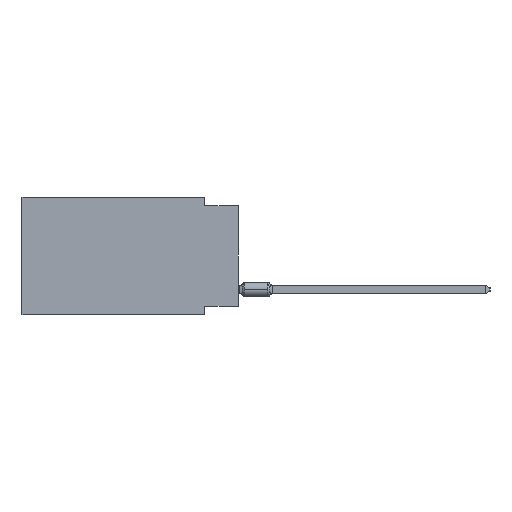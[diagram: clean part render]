
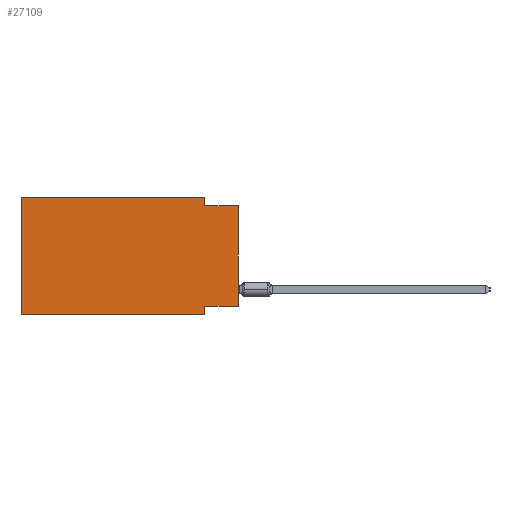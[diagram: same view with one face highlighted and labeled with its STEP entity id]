
A CAD part, left-side view. The second image highlights one B-rep face of the part: STEP entity #27109.
In plain terms, the highlighted planar face has unit normal (-1, 0, 0).
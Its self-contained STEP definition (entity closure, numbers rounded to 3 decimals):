
#609 = CARTESIAN_POINT ( 'NONE',  ( 0., 16.383, 0. ) ) ;
#1250 = LINE ( 'NONE', #60810, #87748 ) ;
#3824 = CARTESIAN_POINT ( 'NONE',  ( 0., 0., -0.635 ) ) ;
#5243 = LINE ( 'NONE', #35043, #7240 ) ;
#6862 = VECTOR ( 'NONE', #86803, 1000. ) ;
#7061 = EDGE_CURVE ( 'NONE', #28672, #7809, #38640, .T. ) ;
#7240 = VECTOR ( 'NONE', #81659, 1000. ) ;
#7387 = VERTEX_POINT ( 'NONE', #59777 ) ;
#7578 = DIRECTION ( 'NONE',  ( 0., 0., 1. ) ) ;
#7809 = VERTEX_POINT ( 'NONE', #36826 ) ;
#8173 = CARTESIAN_POINT ( 'NONE',  ( 0., 2.54, -8.255 ) ) ;
#9667 = LINE ( 'NONE', #47386, #38946 ) ;
#12269 = PLANE ( 'NONE',  #75564 ) ;
#12424 = ORIENTED_EDGE ( 'NONE', *, *, #78448, .F. ) ;
#12964 = VECTOR ( 'NONE', #28660, 1000. ) ;
#13235 = DIRECTION ( 'NONE',  ( 0., 0., -1. ) ) ;
#14143 = VERTEX_POINT ( 'NONE', #71076 ) ;
#15406 = CARTESIAN_POINT ( 'NONE',  ( 0., 2.54, 0. ) ) ;
#16245 = VERTEX_POINT ( 'NONE', #3824 ) ;
#27109 = ADVANCED_FACE ( 'NONE', ( #49978 ), #12269, .F. ) ;
#28228 = ORIENTED_EDGE ( 'NONE', *, *, #65236, .F. ) ;
#28518 = VERTEX_POINT ( 'NONE', #8173 ) ;
#28660 = DIRECTION ( 'NONE',  ( 0., 0., -1. ) ) ;
#28672 = VERTEX_POINT ( 'NONE', #40419 ) ;
#31737 = CARTESIAN_POINT ( 'NONE',  ( 0., 0., -8.255 ) ) ;
#33720 = LINE ( 'NONE', #78874, #6862 ) ;
#35043 = CARTESIAN_POINT ( 'NONE',  ( 0., 16.383, 0. ) ) ;
#36826 = CARTESIAN_POINT ( 'NONE',  ( 0., 2.54, -8.89 ) ) ;
#37214 = EDGE_CURVE ( 'NONE', #7387, #65553, #5243, .T. ) ;
#38640 = LINE ( 'NONE', #75365, #61238 ) ;
#38946 = VECTOR ( 'NONE', #54334, 1000. ) ;
#40171 = EDGE_CURVE ( 'NONE', #65553, #14143, #33720, .T. ) ;
#40419 = CARTESIAN_POINT ( 'NONE',  ( 0., 16.383, -8.89 ) ) ;
#45778 = LINE ( 'NONE', #609, #52050 ) ;
#47386 = CARTESIAN_POINT ( 'NONE',  ( 0., 0., 0. ) ) ;
#49978 = FACE_OUTER_BOUND ( 'NONE', #69047, .T. ) ;
#50135 = VECTOR ( 'NONE', #81292, 1000. ) ;
#52050 = VECTOR ( 'NONE', #7578, 1000. ) ;
#52113 = ORIENTED_EDGE ( 'NONE', *, *, #94581, .F. ) ;
#52591 = EDGE_CURVE ( 'NONE', #75284, #16245, #9667, .T. ) ;
#53855 = DIRECTION ( 'NONE',  ( 0., -1., 0. ) ) ;
#54334 = DIRECTION ( 'NONE',  ( 0., 0., 1. ) ) ;
#54535 = ORIENTED_EDGE ( 'NONE', *, *, #40171, .F. ) ;
#59478 = LINE ( 'NONE', #60924, #50135 ) ;
#59531 = DIRECTION ( 'NONE',  ( 0., -1., 0. ) ) ;
#59777 = CARTESIAN_POINT ( 'NONE',  ( 0., 16.383, 0. ) ) ;
#60810 = CARTESIAN_POINT ( 'NONE',  ( 0., 0., -0.635 ) ) ;
#60924 = CARTESIAN_POINT ( 'NONE',  ( 0., 0., -8.255 ) ) ;
#61238 = VECTOR ( 'NONE', #59531, 1000. ) ;
#65236 = EDGE_CURVE ( 'NONE', #28672, #7387, #45778, .T. ) ;
#65553 = VERTEX_POINT ( 'NONE', #15406 ) ;
#66277 = ORIENTED_EDGE ( 'NONE', *, *, #37214, .F. ) ;
#69047 = EDGE_LOOP ( 'NONE', ( #70773, #12424, #54535, #66277, #28228, #73435, #95441, #52113 ) ) ;
#70773 = ORIENTED_EDGE ( 'NONE', *, *, #52591, .T. ) ;
#71076 = CARTESIAN_POINT ( 'NONE',  ( 0., 2.54, -0.635 ) ) ;
#72801 = DIRECTION ( 'NONE',  ( 1., 0., 0. ) ) ;
#73435 = ORIENTED_EDGE ( 'NONE', *, *, #7061, .T. ) ;
#74771 = EDGE_CURVE ( 'NONE', #28518, #7809, #81739, .T. ) ;
#75284 = VERTEX_POINT ( 'NONE', #31737 ) ;
#75365 = CARTESIAN_POINT ( 'NONE',  ( 0., 16.383, -8.89 ) ) ;
#75564 = AXIS2_PLACEMENT_3D ( 'NONE', #89632, #72801, #13235 ) ;
#78448 = EDGE_CURVE ( 'NONE', #14143, #16245, #1250, .T. ) ;
#78874 = CARTESIAN_POINT ( 'NONE',  ( 0., 2.54, 0. ) ) ;
#81292 = DIRECTION ( 'NONE',  ( 0., 1., 0. ) ) ;
#81659 = DIRECTION ( 'NONE',  ( 0., -1., 0. ) ) ;
#81739 = LINE ( 'NONE', #88683, #12964 ) ;
#86803 = DIRECTION ( 'NONE',  ( 0., 0., -1. ) ) ;
#87748 = VECTOR ( 'NONE', #53855, 1000. ) ;
#88683 = CARTESIAN_POINT ( 'NONE',  ( 0., 2.54, -8.89 ) ) ;
#89632 = CARTESIAN_POINT ( 'NONE',  ( 0., 16.383, 0. ) ) ;
#94581 = EDGE_CURVE ( 'NONE', #75284, #28518, #59478, .T. ) ;
#95441 = ORIENTED_EDGE ( 'NONE', *, *, #74771, .F. ) ;
